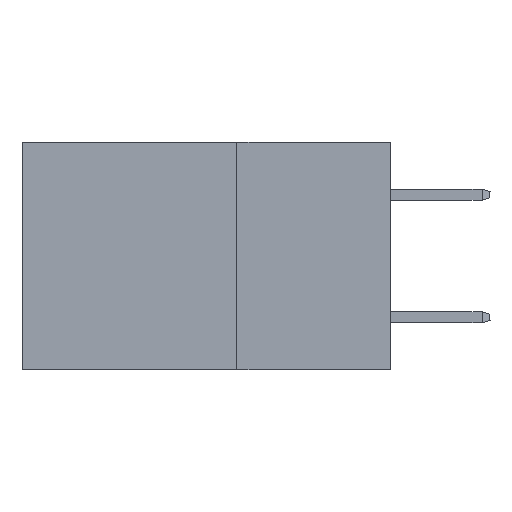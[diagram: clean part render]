
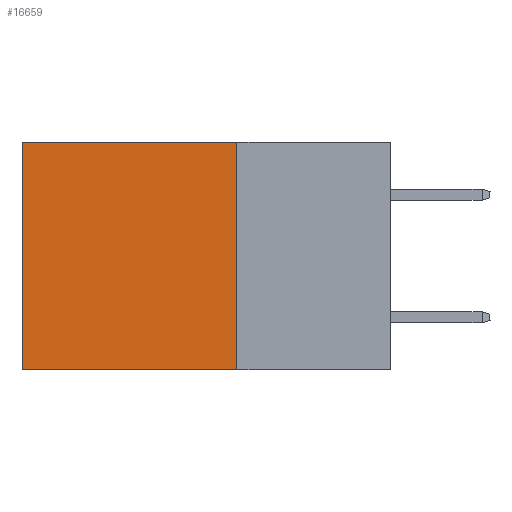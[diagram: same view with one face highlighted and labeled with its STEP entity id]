
A CAD part, left-side view. The second image highlights one B-rep face of the part: STEP entity #16659.
In plain terms, the highlighted planar face has unit normal (-1, 0, 0).
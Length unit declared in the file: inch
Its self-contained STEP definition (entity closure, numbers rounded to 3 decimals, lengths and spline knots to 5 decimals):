
#3970 = VECTOR ( 'NONE', #13284, 39.37008 ) ;
#5840 = ORIENTED_EDGE ( 'NONE', *, *, #16046, .T. ) ;
#6148 = CARTESIAN_POINT ( 'NONE',  ( 0.2875, 0.6, 0. ) ) ;
#6664 = CARTESIAN_POINT ( 'NONE',  ( 0.2875, 0.6, 0. ) ) ;
#9862 = CARTESIAN_POINT ( 'NONE',  ( 0.2875, 0.25, 0. ) ) ;
#10235 = PLANE ( 'NONE',  #18164 ) ;
#10890 = ORIENTED_EDGE ( 'NONE', *, *, #14323, .T. ) ;
#11418 = VERTEX_POINT ( 'NONE', #11932 ) ;
#11573 = FACE_OUTER_BOUND ( 'NONE', #23696, .T. ) ;
#11932 = CARTESIAN_POINT ( 'NONE',  ( 0.2875, 0.6, -0.37 ) ) ;
#12220 = VECTOR ( 'NONE', #25447, 39.37008 ) ;
#12491 = DIRECTION ( 'NONE',  ( 1., 0., 0. ) ) ;
#13284 = DIRECTION ( 'NONE',  ( 0., 0., -1. ) ) ;
#14323 = EDGE_CURVE ( 'NONE', #20249, #11418, #27293, .T. ) ;
#14455 = CARTESIAN_POINT ( 'NONE',  ( 0.2875, 0.25, 0. ) ) ;
#15226 = CARTESIAN_POINT ( 'NONE',  ( 0.2875, 0.25, 0. ) ) ;
#16046 = EDGE_CURVE ( 'NONE', #25126, #20249, #17138, .T. ) ;
#16458 = VECTOR ( 'NONE', #16661, 39.37008 ) ;
#16659 = ADVANCED_FACE ( 'NONE', ( #11573 ), #10235, .F. ) ;
#16661 = DIRECTION ( 'NONE',  ( 0., 1., 0. ) ) ;
#17138 = LINE ( 'NONE', #14455, #16458 ) ;
#17497 = EDGE_CURVE ( 'NONE', #24607, #11418, #18105, .T. ) ;
#18105 = LINE ( 'NONE', #19064, #12220 ) ;
#18164 = AXIS2_PLACEMENT_3D ( 'NONE', #25520, #12491, #27663 ) ;
#18694 = DIRECTION ( 'NONE',  ( 0., 0., -1. ) ) ;
#19064 = CARTESIAN_POINT ( 'NONE',  ( 0.2875, 0.25, -0.37 ) ) ;
#20017 = VECTOR ( 'NONE', #18694, 39.37008 ) ;
#20170 = CARTESIAN_POINT ( 'NONE',  ( 0.2875, 0.25, -0.37 ) ) ;
#20249 = VERTEX_POINT ( 'NONE', #6148 ) ;
#21961 = EDGE_CURVE ( 'NONE', #25126, #24607, #25036, .T. ) ;
#23696 = EDGE_LOOP ( 'NONE', ( #10890, #25057, #24458, #5840 ) ) ;
#24458 = ORIENTED_EDGE ( 'NONE', *, *, #21961, .F. ) ;
#24607 = VERTEX_POINT ( 'NONE', #20170 ) ;
#25036 = LINE ( 'NONE', #9862, #20017 ) ;
#25057 = ORIENTED_EDGE ( 'NONE', *, *, #17497, .F. ) ;
#25126 = VERTEX_POINT ( 'NONE', #15226 ) ;
#25447 = DIRECTION ( 'NONE',  ( 0., 1., 0. ) ) ;
#25520 = CARTESIAN_POINT ( 'NONE',  ( 0.2875, 0.25, 0. ) ) ;
#27293 = LINE ( 'NONE', #6664, #3970 ) ;
#27663 = DIRECTION ( 'NONE',  ( 0., 0., -1. ) ) ;
